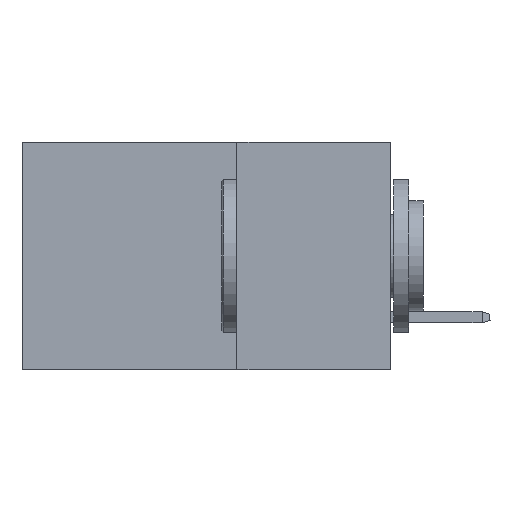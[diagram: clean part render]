
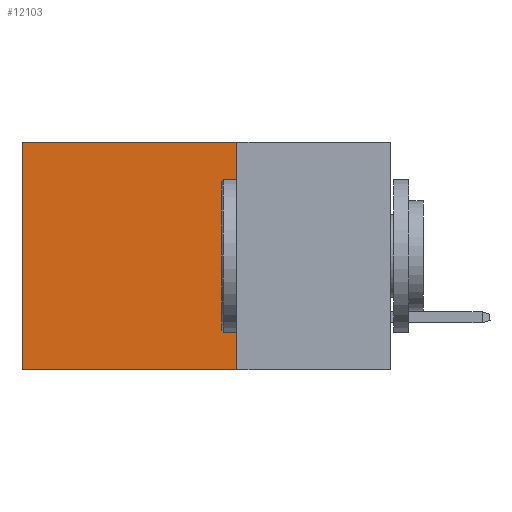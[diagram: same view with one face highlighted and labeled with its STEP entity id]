
A CAD part, left-side view. The second image highlights one B-rep face of the part: STEP entity #12103.
In plain terms, the highlighted planar face has unit normal (-1, 0, 0).
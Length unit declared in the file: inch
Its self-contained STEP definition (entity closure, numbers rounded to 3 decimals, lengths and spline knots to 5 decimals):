
#176 = LINE ( 'NONE', #42077, #25886 ) ;
#1221 = LINE ( 'NONE', #40633, #32190 ) ;
#1730 = VERTEX_POINT ( 'NONE', #40269 ) ;
#2256 = ORIENTED_EDGE ( 'NONE', *, *, #24088, .F. ) ;
#3302 = EDGE_LOOP ( 'NONE', ( #8844, #2256, #4312, #28389 ) ) ;
#3490 = PLANE ( 'NONE',  #16298 ) ;
#3687 = DIRECTION ( 'NONE',  ( 0., 1., 0. ) ) ;
#4312 = ORIENTED_EDGE ( 'NONE', *, *, #22486, .F. ) ;
#4491 = CARTESIAN_POINT ( 'NONE',  ( 0.2875, 0.25, 0. ) ) ;
#7253 = EDGE_CURVE ( 'NONE', #33420, #31298, #41571, .T. ) ;
#8844 = ORIENTED_EDGE ( 'NONE', *, *, #11456, .T. ) ;
#10227 = DIRECTION ( 'NONE',  ( 0., 0., -1. ) ) ;
#11356 = DIRECTION ( 'NONE',  ( 0., 0., -1. ) ) ;
#11456 = EDGE_CURVE ( 'NONE', #31298, #1730, #176, .T. ) ;
#11697 = FACE_OUTER_BOUND ( 'NONE', #3302, .T. ) ;
#11814 = LINE ( 'NONE', #21125, #33794 ) ;
#12103 = ADVANCED_FACE ( 'NONE', ( #11697 ), #3490, .F. ) ;
#14860 = DIRECTION ( 'NONE',  ( 0., 1., 0. ) ) ;
#16298 = AXIS2_PLACEMENT_3D ( 'NONE', #40726, #16657, #10227 ) ;
#16657 = DIRECTION ( 'NONE',  ( 1., 0., 0. ) ) ;
#19942 = DIRECTION ( 'NONE',  ( 0., 0., -1. ) ) ;
#20511 = CARTESIAN_POINT ( 'NONE',  ( 0.2875, 0.6, 0. ) ) ;
#21125 = CARTESIAN_POINT ( 'NONE',  ( 0.2875, 0.25, 0. ) ) ;
#22486 = EDGE_CURVE ( 'NONE', #33420, #37066, #11814, .T. ) ;
#22871 = CARTESIAN_POINT ( 'NONE',  ( 0.2875, 0.25, -0.37 ) ) ;
#24088 = EDGE_CURVE ( 'NONE', #37066, #1730, #1221, .T. ) ;
#25886 = VECTOR ( 'NONE', #19942, 39.37008 ) ;
#28389 = ORIENTED_EDGE ( 'NONE', *, *, #7253, .T. ) ;
#29464 = VECTOR ( 'NONE', #14860, 39.37008 ) ;
#31298 = VERTEX_POINT ( 'NONE', #20511 ) ;
#32190 = VECTOR ( 'NONE', #3687, 39.37008 ) ;
#33420 = VERTEX_POINT ( 'NONE', #41314 ) ;
#33794 = VECTOR ( 'NONE', #11356, 39.37008 ) ;
#37066 = VERTEX_POINT ( 'NONE', #22871 ) ;
#40269 = CARTESIAN_POINT ( 'NONE',  ( 0.2875, 0.6, -0.37 ) ) ;
#40633 = CARTESIAN_POINT ( 'NONE',  ( 0.2875, 0.25, -0.37 ) ) ;
#40726 = CARTESIAN_POINT ( 'NONE',  ( 0.2875, 0.25, 0. ) ) ;
#41314 = CARTESIAN_POINT ( 'NONE',  ( 0.2875, 0.25, 0. ) ) ;
#41571 = LINE ( 'NONE', #4491, #29464 ) ;
#42077 = CARTESIAN_POINT ( 'NONE',  ( 0.2875, 0.6, 0. ) ) ;
